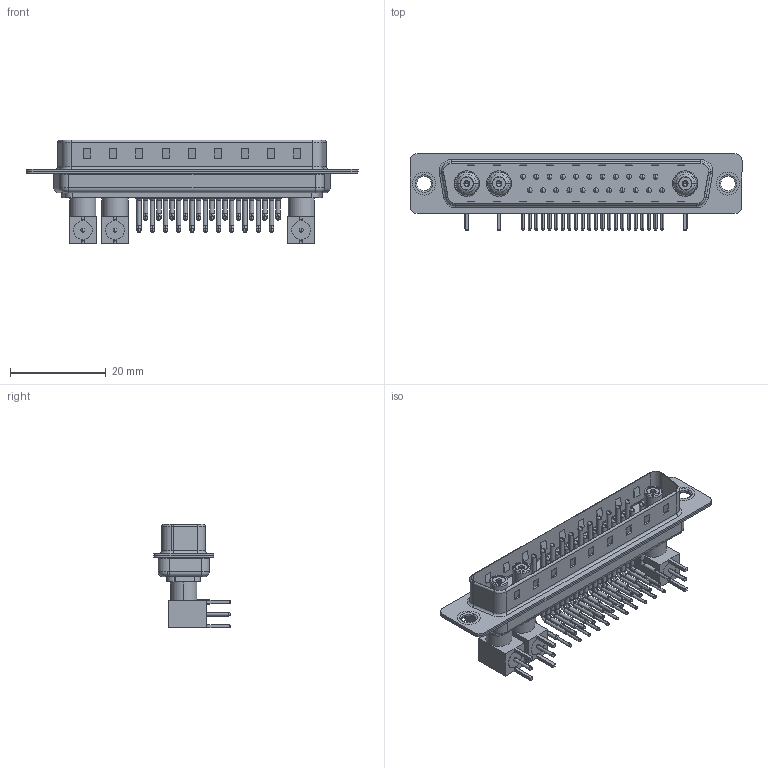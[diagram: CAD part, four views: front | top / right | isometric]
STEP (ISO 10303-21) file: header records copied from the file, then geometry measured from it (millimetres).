
FILE_DESCRIPTION (( 'STEP AP203' ), '1' );
FILE_NAME ('629-25W3640-7N1.STEP', '2022-05-16T09:12:26', ( '' ), ( '' ), 'SwSTEP 2.0', 'SolidWorks 2020', '' );
FILE_SCHEMA (( 'CONFIG_CONTROL_DESIGN' ));
Length unit declared in the file: millimetre
Products named in the file (17): 629Combo Contact Row 2; 629Combo Housing_25W3; 629Combo Shell Rear_37 Contacts; Insulator RA Pin; Co-Ax Jack Assy_RA; 629Combo Thru Hole Rivet; Insulator Socket; Socket_RA; Insulator Socket 2; 629Combo Contact Row 1; Co-Ax Jack_RA PC Tail; 629-25W3640-7N1; RA Back Shell; Locking Collar; 629Combo Shell Front_37 Contacts
Assembly tree (51 placements, depth 3):
  629-25W3640-7N1
    629Combo Housing_25W3
    629Combo Shell Rear_37 Contacts
    629Combo Shell Front_37 Contacts
    629Combo Thru Hole Rivet  x2
    Co-Ax Jack Assy_RA
      Co-Ax Jack_RA PC Tail
      Insulator Socket
      Insulator Socket 2
      Locking Collar
      Socket_RA
      RA Back Shell
      Insulator RA Pin
    Co-Ax Jack Assy_RA
      Co-Ax Jack_RA PC Tail
      Insulator Socket
      Insulator Socket 2
      Locking Collar
      Socket_RA
      RA Back Shell
      Insulator RA Pin
    Co-Ax Jack Assy_RA
      Co-Ax Jack_RA PC Tail
      Insulator Socket
      Insulator Socket 2
      Locking Collar
      Socket_RA
      RA Back Shell
      Insulator RA Pin
    629Combo Contact Row 1  x11
    629Combo Contact Row 2  x11
Bounding box: 69.4 x 16 x 21.71 mm (x, y, z)
Volume: 4725 mm3; surface area: 12601.3 mm2
Topology: 48 solids, 48 shells, 3262 faces, 8852 edges, 5715 vertices
Faces by surface type: plane 1782, cylinder 1118, cone 145, bspline 135, torus 76, sphere 6
Entity records: 30645 total; most frequent: CARTESIAN_POINT 5128, DIRECTION 5029, ORIENTED_EDGE 4532, EDGE_CURVE 2266, AXIS2_PLACEMENT_3D 1844, VERTEX_POINT 1459, LINE 1341, VECTOR 1341
